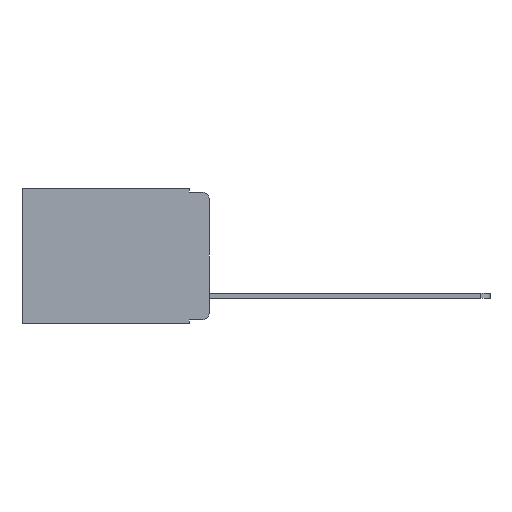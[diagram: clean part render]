
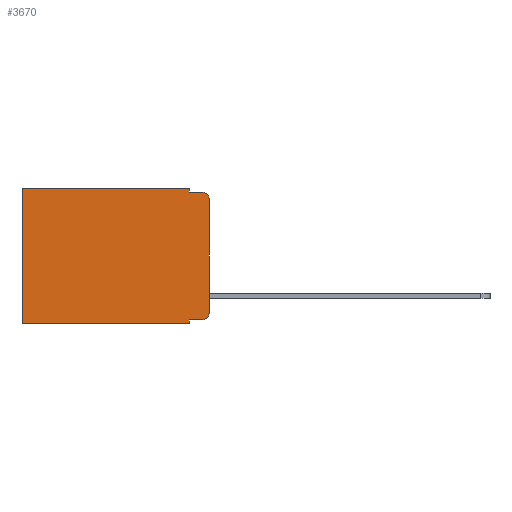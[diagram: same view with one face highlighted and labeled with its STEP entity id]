
A CAD part, left-side view. The second image highlights one B-rep face of the part: STEP entity #3670.
In plain terms, the highlighted planar face has unit normal (-1, 0, 0).
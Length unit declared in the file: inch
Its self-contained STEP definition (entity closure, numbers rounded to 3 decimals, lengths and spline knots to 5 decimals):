
#79 = VECTOR ( 'NONE', #5224, 39.37008 ) ;
#219 = DIRECTION ( 'NONE',  ( 0., -1., 0. ) ) ;
#493 = ORIENTED_EDGE ( 'NONE', *, *, #12664, .F. ) ;
#587 = ORIENTED_EDGE ( 'NONE', *, *, #12975, .T. ) ;
#629 = LINE ( 'NONE', #2314, #8597 ) ;
#798 = ORIENTED_EDGE ( 'NONE', *, *, #9263, .T. ) ;
#878 = ORIENTED_EDGE ( 'NONE', *, *, #6718, .T. ) ;
#976 = LINE ( 'NONE', #9153, #4096 ) ;
#1032 = LINE ( 'NONE', #4348, #1773 ) ;
#1252 = CARTESIAN_POINT ( 'NONE',  ( 0.298, 0.051, -0.01 ) ) ;
#1659 = DIRECTION ( 'NONE',  ( 0., 0., -1. ) ) ;
#1676 = ORIENTED_EDGE ( 'NONE', *, *, #13285, .F. ) ;
#1709 = EDGE_CURVE ( 'NONE', #2611, #7215, #7249, .T. ) ;
#1734 = VECTOR ( 'NONE', #5776, 39.37008 ) ;
#1773 = VECTOR ( 'NONE', #11927, 39.37008 ) ;
#1997 = CARTESIAN_POINT ( 'NONE',  ( 0.298, 0.473, -0.343 ) ) ;
#2043 = ORIENTED_EDGE ( 'NONE', *, *, #4982, .F. ) ;
#2047 = DIRECTION ( 'NONE',  ( 0., 1., 0. ) ) ;
#2113 = CARTESIAN_POINT ( 'NONE',  ( 0.298, 0., 0. ) ) ;
#2314 = CARTESIAN_POINT ( 'NONE',  ( 0.298, 0.051, 0. ) ) ;
#2611 = VERTEX_POINT ( 'NONE', #5650 ) ;
#2712 = DIRECTION ( 'NONE',  ( 0., 0., -1. ) ) ;
#2743 = FACE_OUTER_BOUND ( 'NONE', #5499, .T. ) ;
#2885 = LINE ( 'NONE', #8181, #5844 ) ;
#2999 = CIRCLE ( 'NONE', #7327, 0.02 ) ;
#3258 = CARTESIAN_POINT ( 'NONE',  ( 0.298, 0., -0.343 ) ) ;
#3465 = DIRECTION ( 'NONE',  ( 1., 0., 0. ) ) ;
#3670 = ADVANCED_FACE ( 'NONE', ( #2743 ), #6766, .F. ) ;
#3762 = CARTESIAN_POINT ( 'NONE',  ( 0.298, 0.02, -0.313 ) ) ;
#3961 = VECTOR ( 'NONE', #2047, 39.37008 ) ;
#4096 = VECTOR ( 'NONE', #2712, 39.37008 ) ;
#4348 = CARTESIAN_POINT ( 'NONE',  ( 0.298, 0.051, 0. ) ) ;
#4388 = ORIENTED_EDGE ( 'NONE', *, *, #1709, .T. ) ;
#4547 = AXIS2_PLACEMENT_3D ( 'NONE', #14042, #3465, #9250 ) ;
#4788 = LINE ( 'NONE', #1252, #1734 ) ;
#4982 = EDGE_CURVE ( 'NONE', #7223, #12037, #629, .T. ) ;
#5030 = CARTESIAN_POINT ( 'NONE',  ( 0.298, 0., -0.03 ) ) ;
#5224 = DIRECTION ( 'NONE',  ( 0., 0., -1. ) ) ;
#5499 = EDGE_LOOP ( 'NONE', ( #6096, #10723, #11394, #493, #798, #878, #1676, #2043, #587, #4388 ) ) ;
#5650 = CARTESIAN_POINT ( 'NONE',  ( 0.298, 0.02, -0.333 ) ) ;
#5776 = DIRECTION ( 'NONE',  ( 0., -1., 0. ) ) ;
#5844 = VECTOR ( 'NONE', #219, 39.37008 ) ;
#6096 = ORIENTED_EDGE ( 'NONE', *, *, #12543, .F. ) ;
#6139 = CARTESIAN_POINT ( 'NONE',  ( 0.298, 0.051, -0.01 ) ) ;
#6404 = CARTESIAN_POINT ( 'NONE',  ( 0.298, 0.051, -0.343 ) ) ;
#6630 = EDGE_CURVE ( 'NONE', #9017, #8278, #4788, .T. ) ;
#6718 = EDGE_CURVE ( 'NONE', #7476, #13271, #976, .T. ) ;
#6766 = PLANE ( 'NONE',  #4547 ) ;
#6852 = LINE ( 'NONE', #3258, #3961 ) ;
#7215 = VERTEX_POINT ( 'NONE', #11278 ) ;
#7223 = VERTEX_POINT ( 'NONE', #13382 ) ;
#7249 = CIRCLE ( 'NONE', #8656, 0.02 ) ;
#7327 = AXIS2_PLACEMENT_3D ( 'NONE', #10854, #8366, #1659 ) ;
#7476 = VERTEX_POINT ( 'NONE', #8136 ) ;
#7664 = EDGE_CURVE ( 'NONE', #8462, #8278, #2999, .T. ) ;
#8005 = CARTESIAN_POINT ( 'NONE',  ( 0.298, 0.02, -0.01 ) ) ;
#8136 = CARTESIAN_POINT ( 'NONE',  ( 0.298, 0.473, 0. ) ) ;
#8181 = CARTESIAN_POINT ( 'NONE',  ( 0.298, 0.051, -0.333 ) ) ;
#8278 = VERTEX_POINT ( 'NONE', #8005 ) ;
#8281 = CARTESIAN_POINT ( 'NONE',  ( 0.298, 0.051, 0. ) ) ;
#8366 = DIRECTION ( 'NONE',  ( -1., 0., 0. ) ) ;
#8439 = VERTEX_POINT ( 'NONE', #8281 ) ;
#8462 = VERTEX_POINT ( 'NONE', #5030 ) ;
#8597 = VECTOR ( 'NONE', #13807, 39.37008 ) ;
#8656 = AXIS2_PLACEMENT_3D ( 'NONE', #3762, #9407, #8874 ) ;
#8874 = DIRECTION ( 'NONE',  ( 0., 0., -1. ) ) ;
#9017 = VERTEX_POINT ( 'NONE', #6139 ) ;
#9153 = CARTESIAN_POINT ( 'NONE',  ( 0.298, 0.473, 0. ) ) ;
#9250 = DIRECTION ( 'NONE',  ( 0., 0., -1. ) ) ;
#9263 = EDGE_CURVE ( 'NONE', #8439, #7476, #12939, .T. ) ;
#9407 = DIRECTION ( 'NONE',  ( -1., 0., 0. ) ) ;
#10173 = VECTOR ( 'NONE', #12984, 39.37008 ) ;
#10633 = CARTESIAN_POINT ( 'NONE',  ( 0.298, 0., 0. ) ) ;
#10723 = ORIENTED_EDGE ( 'NONE', *, *, #7664, .T. ) ;
#10854 = CARTESIAN_POINT ( 'NONE',  ( 0.298, 0.02, -0.03 ) ) ;
#11278 = CARTESIAN_POINT ( 'NONE',  ( 0.298, 0., -0.313 ) ) ;
#11394 = ORIENTED_EDGE ( 'NONE', *, *, #6630, .F. ) ;
#11613 = LINE ( 'NONE', #10633, #79 ) ;
#11927 = DIRECTION ( 'NONE',  ( 0., 0., -1. ) ) ;
#12037 = VERTEX_POINT ( 'NONE', #6404 ) ;
#12543 = EDGE_CURVE ( 'NONE', #8462, #7215, #11613, .T. ) ;
#12664 = EDGE_CURVE ( 'NONE', #8439, #9017, #1032, .T. ) ;
#12939 = LINE ( 'NONE', #2113, #10173 ) ;
#12975 = EDGE_CURVE ( 'NONE', #7223, #2611, #2885, .T. ) ;
#12984 = DIRECTION ( 'NONE',  ( 0., 1., 0. ) ) ;
#13271 = VERTEX_POINT ( 'NONE', #1997 ) ;
#13285 = EDGE_CURVE ( 'NONE', #12037, #13271, #6852, .T. ) ;
#13382 = CARTESIAN_POINT ( 'NONE',  ( 0.298, 0.051, -0.333 ) ) ;
#13807 = DIRECTION ( 'NONE',  ( 0., 0., -1. ) ) ;
#14042 = CARTESIAN_POINT ( 'NONE',  ( 0.298, 0., 0. ) ) ;
